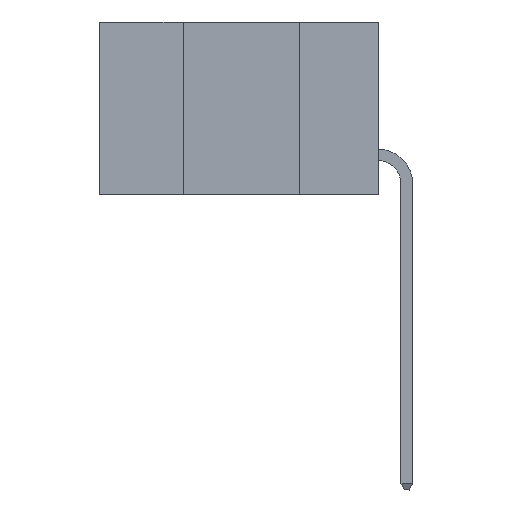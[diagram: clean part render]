
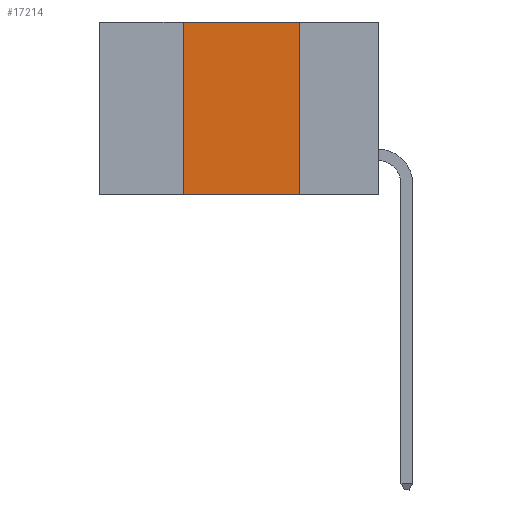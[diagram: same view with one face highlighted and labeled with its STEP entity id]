
A CAD part, left-side view. The second image highlights one B-rep face of the part: STEP entity #17214.
In plain terms, the highlighted planar face has unit normal (-1, 0, 0).
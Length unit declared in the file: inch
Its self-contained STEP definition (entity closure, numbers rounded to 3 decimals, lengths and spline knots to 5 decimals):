
#1309 = CARTESIAN_POINT ( 'NONE',  ( 0., 0.6, 0. ) ) ;
#1821 = ORIENTED_EDGE ( 'NONE', *, *, #17593, .F. ) ;
#1994 = EDGE_LOOP ( 'NONE', ( #1821, #23509, #21860, #21742 ) ) ;
#2389 = VERTEX_POINT ( 'NONE', #18312 ) ;
#2500 = DIRECTION ( 'NONE',  ( 0., 0., 1. ) ) ;
#2969 = EDGE_CURVE ( 'NONE', #12109, #23548, #18971, .T. ) ;
#3077 = AXIS2_PLACEMENT_3D ( 'NONE', #1309, #7807, #22778 ) ;
#4700 = VECTOR ( 'NONE', #23923, 39.37008 ) ;
#6382 = CARTESIAN_POINT ( 'NONE',  ( 0., 0.42, -0.37 ) ) ;
#6829 = CARTESIAN_POINT ( 'NONE',  ( 0., 0.42, 0. ) ) ;
#6834 = CARTESIAN_POINT ( 'NONE',  ( 0., 0.17, 0. ) ) ;
#7233 = DIRECTION ( 'NONE',  ( 0., -1., 0. ) ) ;
#7807 = DIRECTION ( 'NONE',  ( 1., 0., 0. ) ) ;
#8482 = CARTESIAN_POINT ( 'NONE',  ( 0., 0.17, 0. ) ) ;
#9299 = EDGE_CURVE ( 'NONE', #12109, #2389, #11800, .T. ) ;
#11800 = LINE ( 'NONE', #6829, #17535 ) ;
#12071 = VERTEX_POINT ( 'NONE', #8482 ) ;
#12109 = VERTEX_POINT ( 'NONE', #6382 ) ;
#13667 = CARTESIAN_POINT ( 'NONE',  ( 0., 0.6, -0.37 ) ) ;
#14230 = PLANE ( 'NONE',  #3077 ) ;
#14846 = FACE_OUTER_BOUND ( 'NONE', #1994, .T. ) ;
#15467 = VECTOR ( 'NONE', #22765, 39.37008 ) ;
#16390 = CARTESIAN_POINT ( 'NONE',  ( 0., 0.6, 0. ) ) ;
#17214 = ADVANCED_FACE ( 'NONE', ( #14846 ), #14230, .F. ) ;
#17408 = CARTESIAN_POINT ( 'NONE',  ( 0., 0.17, -0.37 ) ) ;
#17535 = VECTOR ( 'NONE', #2500, 39.37008 ) ;
#17593 = EDGE_CURVE ( 'NONE', #12071, #23548, #21808, .T. ) ;
#18312 = CARTESIAN_POINT ( 'NONE',  ( 0., 0.42, 0. ) ) ;
#18971 = LINE ( 'NONE', #13667, #23868 ) ;
#21742 = ORIENTED_EDGE ( 'NONE', *, *, #2969, .T. ) ;
#21808 = LINE ( 'NONE', #6834, #4700 ) ;
#21860 = ORIENTED_EDGE ( 'NONE', *, *, #9299, .F. ) ;
#22765 = DIRECTION ( 'NONE',  ( 0., -1., 0. ) ) ;
#22778 = DIRECTION ( 'NONE',  ( 0., 0., -1. ) ) ;
#23509 = ORIENTED_EDGE ( 'NONE', *, *, #26237, .F. ) ;
#23548 = VERTEX_POINT ( 'NONE', #17408 ) ;
#23868 = VECTOR ( 'NONE', #7233, 39.37008 ) ;
#23923 = DIRECTION ( 'NONE',  ( 0., 0., -1. ) ) ;
#26237 = EDGE_CURVE ( 'NONE', #2389, #12071, #27388, .T. ) ;
#27388 = LINE ( 'NONE', #16390, #15467 ) ;
